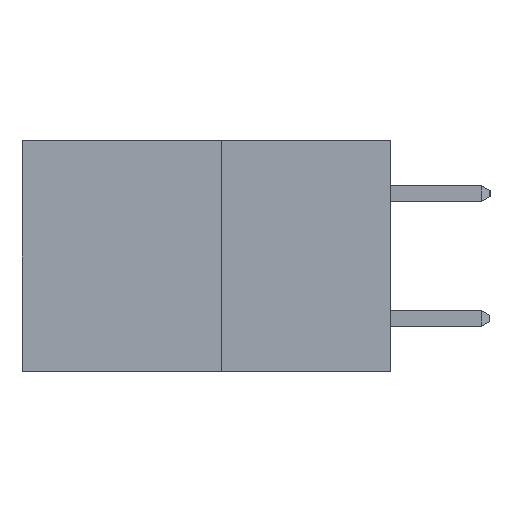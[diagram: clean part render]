
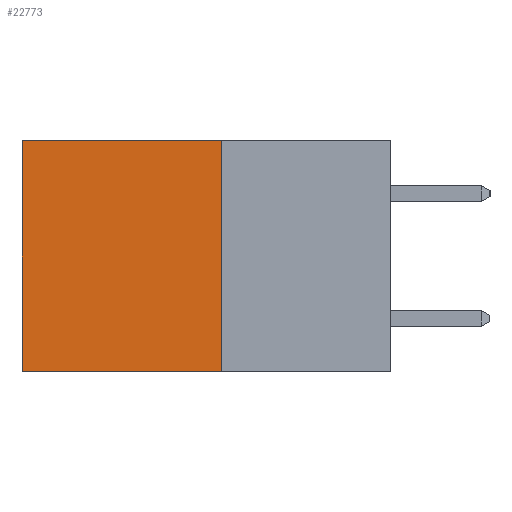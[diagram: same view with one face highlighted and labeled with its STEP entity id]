
A CAD part, left-side view. The second image highlights one B-rep face of the part: STEP entity #22773.
In plain terms, the highlighted planar face has unit normal (-1, 0, 0).
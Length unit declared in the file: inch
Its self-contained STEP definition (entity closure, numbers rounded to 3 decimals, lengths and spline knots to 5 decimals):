
#445 = CARTESIAN_POINT ( 'NONE',  ( 0.277, 0.27, 0. ) ) ;
#836 = CARTESIAN_POINT ( 'NONE',  ( 0.277, 0.59, -0.37 ) ) ;
#963 = CARTESIAN_POINT ( 'NONE',  ( 0.277, 0.27, -0.37 ) ) ;
#1359 = VERTEX_POINT ( 'NONE', #8267 ) ;
#2768 = DIRECTION ( 'NONE',  ( 0., 1., 0. ) ) ;
#3154 = DIRECTION ( 'NONE',  ( 0., 0., -1. ) ) ;
#3371 = DIRECTION ( 'NONE',  ( 1., 0., 0. ) ) ;
#3474 = VECTOR ( 'NONE', #7440, 39.37008 ) ;
#4705 = AXIS2_PLACEMENT_3D ( 'NONE', #963, #3371, #19809 ) ;
#5090 = CARTESIAN_POINT ( 'NONE',  ( 0.277, 0.27, -0.37 ) ) ;
#6273 = EDGE_CURVE ( 'NONE', #22966, #1359, #8607, .T. ) ;
#6467 = EDGE_CURVE ( 'NONE', #1359, #16034, #22206, .T. ) ;
#7279 = LINE ( 'NONE', #445, #12819 ) ;
#7440 = DIRECTION ( 'NONE',  ( 0., 1., 0. ) ) ;
#8147 = VERTEX_POINT ( 'NONE', #11904 ) ;
#8267 = CARTESIAN_POINT ( 'NONE',  ( 0.277, 0.27, -0.37 ) ) ;
#8607 = LINE ( 'NONE', #9223, #14890 ) ;
#9023 = EDGE_CURVE ( 'NONE', #8147, #16034, #23413, .T. ) ;
#9223 = CARTESIAN_POINT ( 'NONE',  ( 0.277, 0.27, -0.37 ) ) ;
#10116 = ORIENTED_EDGE ( 'NONE', *, *, #6273, .F. ) ;
#10942 = CARTESIAN_POINT ( 'NONE',  ( 0.277, 0.27, 0. ) ) ;
#11904 = CARTESIAN_POINT ( 'NONE',  ( 0.277, 0.59, 0. ) ) ;
#12712 = PLANE ( 'NONE',  #4705 ) ;
#12819 = VECTOR ( 'NONE', #2768, 39.37008 ) ;
#13952 = DIRECTION ( 'NONE',  ( 0., 0., -1. ) ) ;
#14574 = FACE_OUTER_BOUND ( 'NONE', #18974, .T. ) ;
#14890 = VECTOR ( 'NONE', #13952, 39.37008 ) ;
#14946 = ORIENTED_EDGE ( 'NONE', *, *, #9023, .T. ) ;
#16034 = VERTEX_POINT ( 'NONE', #24529 ) ;
#18974 = EDGE_LOOP ( 'NONE', ( #14946, #20494, #10116, #27915 ) ) ;
#19809 = DIRECTION ( 'NONE',  ( 0., 0., -1. ) ) ;
#20494 = ORIENTED_EDGE ( 'NONE', *, *, #6467, .F. ) ;
#20564 = EDGE_CURVE ( 'NONE', #22966, #8147, #7279, .T. ) ;
#22206 = LINE ( 'NONE', #5090, #3474 ) ;
#22773 = ADVANCED_FACE ( 'NONE', ( #14574 ), #12712, .F. ) ;
#22966 = VERTEX_POINT ( 'NONE', #10942 ) ;
#23413 = LINE ( 'NONE', #836, #28131 ) ;
#24529 = CARTESIAN_POINT ( 'NONE',  ( 0.277, 0.59, -0.37 ) ) ;
#27915 = ORIENTED_EDGE ( 'NONE', *, *, #20564, .T. ) ;
#28131 = VECTOR ( 'NONE', #3154, 39.37008 ) ;
